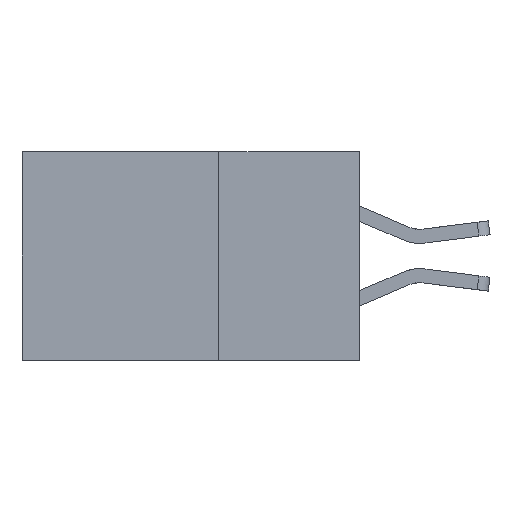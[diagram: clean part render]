
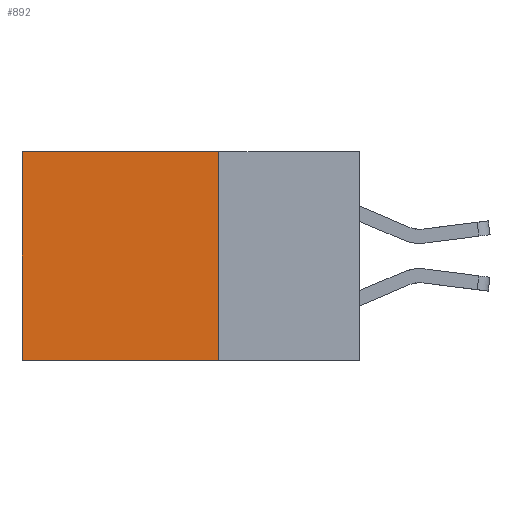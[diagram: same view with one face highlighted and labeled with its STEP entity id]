
A CAD part, left-side view. The second image highlights one B-rep face of the part: STEP entity #892.
In plain terms, the highlighted planar face has unit normal (-1, 0, 0).
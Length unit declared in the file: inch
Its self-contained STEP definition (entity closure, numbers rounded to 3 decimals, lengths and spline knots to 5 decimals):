
#276 = CARTESIAN_POINT ( 'NONE',  ( 0.2875, 0.6, -0.37 ) ) ;
#572 = VERTEX_POINT ( 'NONE', #8306 ) ;
#764 = DIRECTION ( 'NONE',  ( 0., 0., -1. ) ) ;
#783 = CARTESIAN_POINT ( 'NONE',  ( 0.2875, 0.25, 0. ) ) ;
#888 = AXIS2_PLACEMENT_3D ( 'NONE', #783, #948, #764 ) ;
#892 = ADVANCED_FACE ( 'NONE', ( #10385 ), #5094, .F. ) ;
#948 = DIRECTION ( 'NONE',  ( 1., 0., 0. ) ) ;
#1598 = LINE ( 'NONE', #14769, #10513 ) ;
#1772 = LINE ( 'NONE', #7076, #10328 ) ;
#1785 = VERTEX_POINT ( 'NONE', #276 ) ;
#2318 = DIRECTION ( 'NONE',  ( 0., 0., -1. ) ) ;
#3283 = EDGE_CURVE ( 'NONE', #8737, #1785, #1772, .T. ) ;
#4058 = EDGE_CURVE ( 'NONE', #572, #1785, #8661, .T. ) ;
#4184 = CARTESIAN_POINT ( 'NONE',  ( 0.2875, 0.25, -0.37 ) ) ;
#4673 = CARTESIAN_POINT ( 'NONE',  ( 0.2875, 0.25, 0. ) ) ;
#4681 = CARTESIAN_POINT ( 'NONE',  ( 0.2875, 0.6, 0. ) ) ;
#5083 = VERTEX_POINT ( 'NONE', #14111 ) ;
#5094 = PLANE ( 'NONE',  #888 ) ;
#7076 = CARTESIAN_POINT ( 'NONE',  ( 0.2875, 0.25, -0.37 ) ) ;
#8306 = CARTESIAN_POINT ( 'NONE',  ( 0.2875, 0.6, 0. ) ) ;
#8661 = LINE ( 'NONE', #4681, #14207 ) ;
#8737 = VERTEX_POINT ( 'NONE', #4184 ) ;
#9613 = DIRECTION ( 'NONE',  ( 0., 1., 0. ) ) ;
#9658 = EDGE_CURVE ( 'NONE', #5083, #572, #13465, .T. ) ;
#10047 = DIRECTION ( 'NONE',  ( 0., 0., -1. ) ) ;
#10296 = VECTOR ( 'NONE', #9613, 39.37008 ) ;
#10328 = VECTOR ( 'NONE', #15381, 39.37008 ) ;
#10385 = FACE_OUTER_BOUND ( 'NONE', #13530, .T. ) ;
#10513 = VECTOR ( 'NONE', #10047, 39.37008 ) ;
#11256 = ORIENTED_EDGE ( 'NONE', *, *, #3283, .F. ) ;
#11638 = ORIENTED_EDGE ( 'NONE', *, *, #15079, .F. ) ;
#13465 = LINE ( 'NONE', #4673, #10296 ) ;
#13530 = EDGE_LOOP ( 'NONE', ( #13680, #11256, #11638, #14791 ) ) ;
#13680 = ORIENTED_EDGE ( 'NONE', *, *, #4058, .T. ) ;
#14111 = CARTESIAN_POINT ( 'NONE',  ( 0.2875, 0.25, 0. ) ) ;
#14207 = VECTOR ( 'NONE', #2318, 39.37008 ) ;
#14769 = CARTESIAN_POINT ( 'NONE',  ( 0.2875, 0.25, 0. ) ) ;
#14791 = ORIENTED_EDGE ( 'NONE', *, *, #9658, .T. ) ;
#15079 = EDGE_CURVE ( 'NONE', #5083, #8737, #1598, .T. ) ;
#15381 = DIRECTION ( 'NONE',  ( 0., 1., 0. ) ) ;
